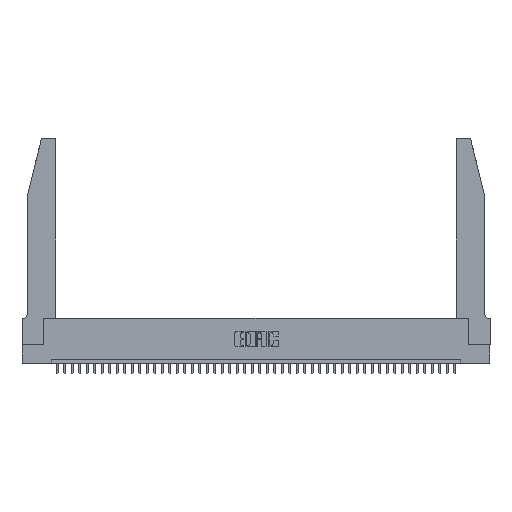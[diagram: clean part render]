
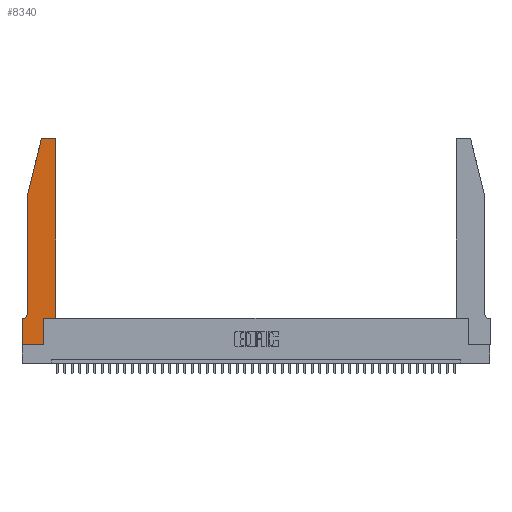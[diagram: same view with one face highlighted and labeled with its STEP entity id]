
A CAD part, top view. The second image highlights one B-rep face of the part: STEP entity #8340.
In plain terms, the highlighted planar face has unit normal (0, 0, 1).
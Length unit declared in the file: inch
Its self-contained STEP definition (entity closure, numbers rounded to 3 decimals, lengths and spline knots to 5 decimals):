
#180 = AXIS2_PLACEMENT_3D ( 'NONE', #18504, #9623, #13048 ) ;
#705 = VECTOR ( 'NONE', #19303, 39.37008 ) ;
#1638 = LINE ( 'NONE', #12226, #14359 ) ;
#2000 = CARTESIAN_POINT ( 'NONE',  ( 0.0755, 2., 0.37 ) ) ;
#2809 = EDGE_CURVE ( 'NONE', #3184, #8116, #10435, .T. ) ;
#2982 = CARTESIAN_POINT ( 'NONE',  ( 0.4205, 2.75, 0.37 ) ) ;
#3142 = ORIENTED_EDGE ( 'NONE', *, *, #3899, .T. ) ;
#3184 = VERTEX_POINT ( 'NONE', #2982 ) ;
#3290 = VERTEX_POINT ( 'NONE', #13443 ) ;
#3581 = EDGE_CURVE ( 'NONE', #17756, #16141, #29925, .T. ) ;
#3899 = EDGE_CURVE ( 'NONE', #39687, #18425, #27232, .T. ) ;
#4442 = DIRECTION ( 'NONE',  ( 1., 0., 0. ) ) ;
#4658 = CARTESIAN_POINT ( 'NONE',  ( 0.4505, 0.35, 0.37 ) ) ;
#4885 = ORIENTED_EDGE ( 'NONE', *, *, #41437, .T. ) ;
#5661 = ORIENTED_EDGE ( 'NONE', *, *, #8742, .T. ) ;
#6480 = LINE ( 'NONE', #36654, #37653 ) ;
#6788 = DIRECTION ( 'NONE',  ( -1., 0., 0. ) ) ;
#7696 = DIRECTION ( 'NONE',  ( 0., 0., 1. ) ) ;
#7697 = LINE ( 'NONE', #4658, #33629 ) ;
#8114 = CARTESIAN_POINT ( 'NONE',  ( 0.0755, 0.35, 0.37 ) ) ;
#8116 = VERTEX_POINT ( 'NONE', #28290 ) ;
#8340 = ADVANCED_FACE ( 'NONE', ( #28164 ), #23494, .T. ) ;
#8493 = EDGE_CURVE ( 'NONE', #18425, #41634, #38187, .T. ) ;
#8742 = EDGE_CURVE ( 'NONE', #23509, #17756, #6480, .T. ) ;
#9191 = LINE ( 'NONE', #2000, #705 ) ;
#9423 = CARTESIAN_POINT ( 'NONE',  ( 0.4505, 0.35, 0.37 ) ) ;
#9623 = DIRECTION ( 'NONE',  ( 0., 0., 1. ) ) ;
#10435 = LINE ( 'NONE', #43666, #39529 ) ;
#10782 = EDGE_CURVE ( 'NONE', #16714, #3184, #13257, .T. ) ;
#12226 = CARTESIAN_POINT ( 'NONE',  ( 0.2865, 0.35, 0.37 ) ) ;
#12386 = DIRECTION ( 'NONE',  ( 0., 1., 0. ) ) ;
#13048 = DIRECTION ( 'NONE',  ( 1., 0., 0. ) ) ;
#13254 = EDGE_CURVE ( 'NONE', #39467, #16714, #7697, .T. ) ;
#13257 = CIRCLE ( 'NONE', #26878, 0.03 ) ;
#13443 = CARTESIAN_POINT ( 'NONE',  ( 0.2865, 0.35, 0.37 ) ) ;
#13520 = EDGE_LOOP ( 'NONE', ( #21987, #25476, #20479, #3142, #28635, #35778, #5661, #18689, #4885, #15136, #33357, #26616 ) ) ;
#13710 = CARTESIAN_POINT ( 'NONE',  ( 0.4505, 0.35, 0.37 ) ) ;
#13735 = CARTESIAN_POINT ( 'NONE',  ( 0.0755, 2., 0.37 ) ) ;
#14135 = DIRECTION ( 'NONE',  ( 1., 0., 0. ) ) ;
#14359 = VECTOR ( 'NONE', #12386, 39.37008 ) ;
#15136 = ORIENTED_EDGE ( 'NONE', *, *, #28406, .T. ) ;
#16141 = VERTEX_POINT ( 'NONE', #35834 ) ;
#16356 = CARTESIAN_POINT ( 'NONE',  ( 0.0755, 2., 0.37 ) ) ;
#16714 = VERTEX_POINT ( 'NONE', #42859 ) ;
#17756 = VERTEX_POINT ( 'NONE', #24179 ) ;
#18425 = VERTEX_POINT ( 'NONE', #39193 ) ;
#18504 = CARTESIAN_POINT ( 'NONE',  ( 0., 0.35, 0.37 ) ) ;
#18689 = ORIENTED_EDGE ( 'NONE', *, *, #3581, .T. ) ;
#19303 = DIRECTION ( 'NONE',  ( -0.239, -0.971, 0. ) ) ;
#20479 = ORIENTED_EDGE ( 'NONE', *, *, #21679, .T. ) ;
#20904 = VECTOR ( 'NONE', #36306, 39.37008 ) ;
#21679 = EDGE_CURVE ( 'NONE', #24266, #39687, #9191, .T. ) ;
#21987 = ORIENTED_EDGE ( 'NONE', *, *, #2809, .T. ) ;
#23318 = CARTESIAN_POINT ( 'NONE',  ( 0., 0.35, 0.37 ) ) ;
#23494 = PLANE ( 'NONE',  #180 ) ;
#23509 = VERTEX_POINT ( 'NONE', #23318 ) ;
#23649 = CARTESIAN_POINT ( 'NONE',  ( 0.0055, 0.42, 0.37 ) ) ;
#24179 = CARTESIAN_POINT ( 'NONE',  ( 0., 0., 0.37 ) ) ;
#24266 = VERTEX_POINT ( 'NONE', #34144 ) ;
#24859 = VECTOR ( 'NONE', #28509, 39.37008 ) ;
#25399 = LINE ( 'NONE', #8114, #24859 ) ;
#25476 = ORIENTED_EDGE ( 'NONE', *, *, #29625, .T. ) ;
#25665 = VECTOR ( 'NONE', #30868, 39.37008 ) ;
#26143 = CARTESIAN_POINT ( 'NONE',  ( 0., 0., 0.37 ) ) ;
#26486 = AXIS2_PLACEMENT_3D ( 'NONE', #27939, #7696, #4442 ) ;
#26616 = ORIENTED_EDGE ( 'NONE', *, *, #10782, .T. ) ;
#26632 = DIRECTION ( 'NONE',  ( 1., 0., 0. ) ) ;
#26878 = AXIS2_PLACEMENT_3D ( 'NONE', #42876, #36500, #26632 ) ;
#27039 = DIRECTION ( 'NONE',  ( 0., 0., -1. ) ) ;
#27232 = LINE ( 'NONE', #13735, #25665 ) ;
#27939 = CARTESIAN_POINT ( 'NONE',  ( 0.284, 2.72, 0.37 ) ) ;
#28164 = FACE_OUTER_BOUND ( 'NONE', #13520, .T. ) ;
#28278 = LINE ( 'NONE', #13710, #38310 ) ;
#28290 = CARTESIAN_POINT ( 'NONE',  ( 0.284, 2.75, 0.37 ) ) ;
#28406 = EDGE_CURVE ( 'NONE', #3290, #39467, #28278, .T. ) ;
#28509 = DIRECTION ( 'NONE',  ( -1., 0., 0. ) ) ;
#28635 = ORIENTED_EDGE ( 'NONE', *, *, #8493, .T. ) ;
#29625 = EDGE_CURVE ( 'NONE', #8116, #24266, #41438, .T. ) ;
#29925 = LINE ( 'NONE', #26143, #20904 ) ;
#30868 = DIRECTION ( 'NONE',  ( 0., -1., 0. ) ) ;
#33357 = ORIENTED_EDGE ( 'NONE', *, *, #13254, .T. ) ;
#33629 = VECTOR ( 'NONE', #35240, 39.37008 ) ;
#33900 = DIRECTION ( 'NONE',  ( -1., 0., 0. ) ) ;
#34144 = CARTESIAN_POINT ( 'NONE',  ( 0.25487, 2.72718, 0.37 ) ) ;
#35240 = DIRECTION ( 'NONE',  ( 0., 1., 0. ) ) ;
#35778 = ORIENTED_EDGE ( 'NONE', *, *, #42540, .T. ) ;
#35834 = CARTESIAN_POINT ( 'NONE',  ( 0.2865, 0., 0.37 ) ) ;
#36306 = DIRECTION ( 'NONE',  ( 1., 0., 0. ) ) ;
#36500 = DIRECTION ( 'NONE',  ( 0., 0., 1. ) ) ;
#36654 = CARTESIAN_POINT ( 'NONE',  ( 0., 0., 0.37 ) ) ;
#37653 = VECTOR ( 'NONE', #43024, 39.37008 ) ;
#38081 = AXIS2_PLACEMENT_3D ( 'NONE', #23649, #27039, #6788 ) ;
#38187 = CIRCLE ( 'NONE', #38081, 0.07 ) ;
#38310 = VECTOR ( 'NONE', #14135, 39.37008 ) ;
#39193 = CARTESIAN_POINT ( 'NONE',  ( 0.0755, 0.42, 0.37 ) ) ;
#39467 = VERTEX_POINT ( 'NONE', #9423 ) ;
#39529 = VECTOR ( 'NONE', #33900, 39.37008 ) ;
#39687 = VERTEX_POINT ( 'NONE', #16356 ) ;
#40566 = CARTESIAN_POINT ( 'NONE',  ( 0.0055, 0.35, 0.37 ) ) ;
#41437 = EDGE_CURVE ( 'NONE', #16141, #3290, #1638, .T. ) ;
#41438 = CIRCLE ( 'NONE', #26486, 0.03 ) ;
#41634 = VERTEX_POINT ( 'NONE', #40566 ) ;
#42540 = EDGE_CURVE ( 'NONE', #41634, #23509, #25399, .T. ) ;
#42859 = CARTESIAN_POINT ( 'NONE',  ( 0.4505, 2.72, 0.37 ) ) ;
#42876 = CARTESIAN_POINT ( 'NONE',  ( 0.4205, 2.72, 0.37 ) ) ;
#43024 = DIRECTION ( 'NONE',  ( 0., -1., 0. ) ) ;
#43666 = CARTESIAN_POINT ( 'NONE',  ( 0.2605, 2.75, 0.37 ) ) ;
